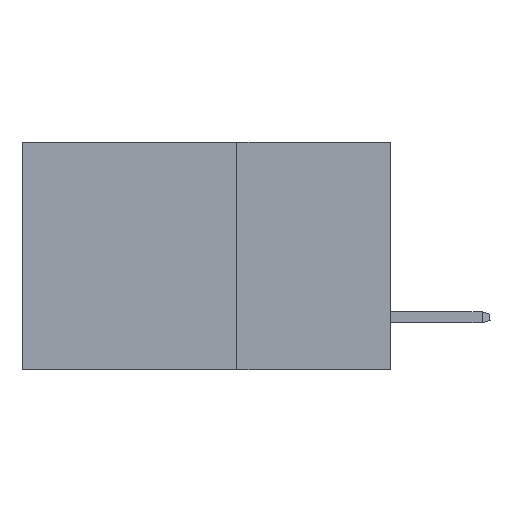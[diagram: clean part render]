
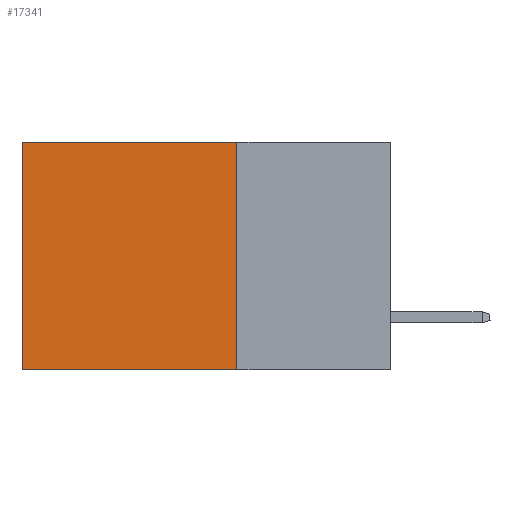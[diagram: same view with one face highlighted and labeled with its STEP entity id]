
A CAD part, left-side view. The second image highlights one B-rep face of the part: STEP entity #17341.
In plain terms, the highlighted planar face has unit normal (-1, 0, 0).
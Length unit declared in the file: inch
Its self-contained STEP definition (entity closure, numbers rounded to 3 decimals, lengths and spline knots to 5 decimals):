
#352 = CARTESIAN_POINT ( 'NONE',  ( 0.2875, 0.6, 0. ) ) ;
#557 = AXIS2_PLACEMENT_3D ( 'NONE', #1555, #15742, #25642 ) ;
#763 = CARTESIAN_POINT ( 'NONE',  ( 0.2875, 0.25, 0. ) ) ;
#881 = DIRECTION ( 'NONE',  ( 0., 1., 0. ) ) ;
#1055 = EDGE_LOOP ( 'NONE', ( #23483, #1592, #19440, #14712 ) ) ;
#1555 = CARTESIAN_POINT ( 'NONE',  ( 0.2875, 0.25, 0. ) ) ;
#1592 = ORIENTED_EDGE ( 'NONE', *, *, #13463, .F. ) ;
#3053 = VECTOR ( 'NONE', #9377, 39.37008 ) ;
#4268 = LINE ( 'NONE', #19142, #4585 ) ;
#4585 = VECTOR ( 'NONE', #881, 39.37008 ) ;
#5795 = EDGE_CURVE ( 'NONE', #23647, #18801, #7838, .T. ) ;
#6744 = CARTESIAN_POINT ( 'NONE',  ( 0.2875, 0.25, -0.37 ) ) ;
#7135 = LINE ( 'NONE', #6744, #20399 ) ;
#7227 = DIRECTION ( 'NONE',  ( 0., 1., 0. ) ) ;
#7838 = LINE ( 'NONE', #11733, #17628 ) ;
#9377 = DIRECTION ( 'NONE',  ( 0., 0., -1. ) ) ;
#11733 = CARTESIAN_POINT ( 'NONE',  ( 0.2875, 0.6, 0. ) ) ;
#13463 = EDGE_CURVE ( 'NONE', #22981, #18801, #7135, .T. ) ;
#13590 = DIRECTION ( 'NONE',  ( 0., 0., -1. ) ) ;
#13601 = EDGE_CURVE ( 'NONE', #19931, #23647, #4268, .T. ) ;
#13887 = PLANE ( 'NONE',  #557 ) ;
#14712 = ORIENTED_EDGE ( 'NONE', *, *, #13601, .T. ) ;
#15742 = DIRECTION ( 'NONE',  ( 1., 0., 0. ) ) ;
#16520 = CARTESIAN_POINT ( 'NONE',  ( 0.2875, 0.6, -0.37 ) ) ;
#16619 = EDGE_CURVE ( 'NONE', #19931, #22981, #19165, .T. ) ;
#17341 = ADVANCED_FACE ( 'NONE', ( #19117 ), #13887, .F. ) ;
#17628 = VECTOR ( 'NONE', #13590, 39.37008 ) ;
#18801 = VERTEX_POINT ( 'NONE', #16520 ) ;
#19117 = FACE_OUTER_BOUND ( 'NONE', #1055, .T. ) ;
#19142 = CARTESIAN_POINT ( 'NONE',  ( 0.2875, 0.25, 0. ) ) ;
#19165 = LINE ( 'NONE', #25387, #3053 ) ;
#19440 = ORIENTED_EDGE ( 'NONE', *, *, #16619, .F. ) ;
#19931 = VERTEX_POINT ( 'NONE', #763 ) ;
#20399 = VECTOR ( 'NONE', #7227, 39.37008 ) ;
#22981 = VERTEX_POINT ( 'NONE', #25444 ) ;
#23483 = ORIENTED_EDGE ( 'NONE', *, *, #5795, .T. ) ;
#23647 = VERTEX_POINT ( 'NONE', #352 ) ;
#25387 = CARTESIAN_POINT ( 'NONE',  ( 0.2875, 0.25, 0. ) ) ;
#25444 = CARTESIAN_POINT ( 'NONE',  ( 0.2875, 0.25, -0.37 ) ) ;
#25642 = DIRECTION ( 'NONE',  ( 0., 0., -1. ) ) ;
